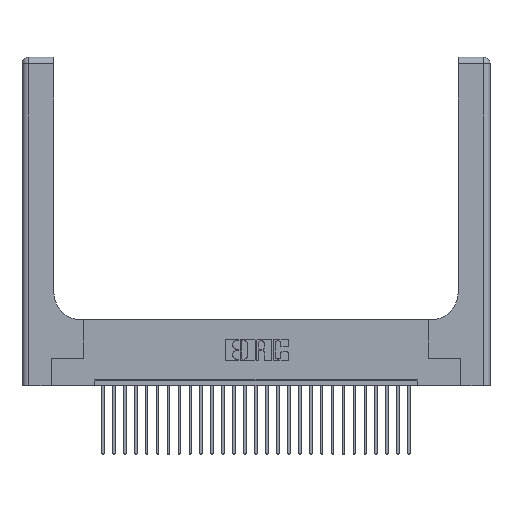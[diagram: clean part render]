
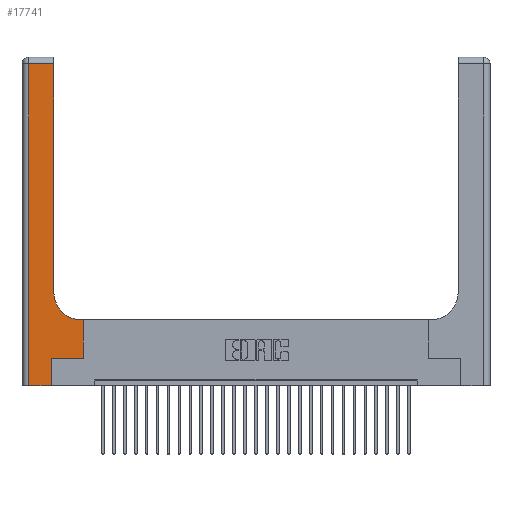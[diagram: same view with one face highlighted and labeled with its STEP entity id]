
A CAD part, top view. The second image highlights one B-rep face of the part: STEP entity #17741.
In plain terms, the highlighted planar face has unit normal (0, 0, 1).
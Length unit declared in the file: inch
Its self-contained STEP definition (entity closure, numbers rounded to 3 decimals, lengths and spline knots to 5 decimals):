
#417 = DIRECTION ( 'NONE',  ( -1., 0., 0. ) ) ;
#625 = PLANE ( 'NONE',  #6170 ) ;
#840 = CARTESIAN_POINT ( 'NONE',  ( 0.269, 0., 0.37 ) ) ;
#1347 = EDGE_LOOP ( 'NONE', ( #9175, #4184, #26375, #19203, #22407, #16420, #15048, #18807, #2289 ) ) ;
#1500 = AXIS2_PLACEMENT_3D ( 'NONE', #2193, #4414, #19921 ) ;
#2193 = CARTESIAN_POINT ( 'NONE',  ( 0.5415, 0.85, 0.37 ) ) ;
#2289 = ORIENTED_EDGE ( 'NONE', *, *, #15588, .T. ) ;
#2586 = CARTESIAN_POINT ( 'NONE',  ( 0.2915, 3., 0.37 ) ) ;
#2830 = VERTEX_POINT ( 'NONE', #20505 ) ;
#2966 = DIRECTION ( 'NONE',  ( 0., 1., 0. ) ) ;
#3234 = VECTOR ( 'NONE', #13790, 39.37008 ) ;
#3488 = VERTEX_POINT ( 'NONE', #12403 ) ;
#3917 = LINE ( 'NONE', #2586, #25105 ) ;
#4184 = ORIENTED_EDGE ( 'NONE', *, *, #13739, .T. ) ;
#4414 = DIRECTION ( 'NONE',  ( 0., 0., -1. ) ) ;
#4585 = CARTESIAN_POINT ( 'NONE',  ( 0.5585, 0.25, 0.37 ) ) ;
#4624 = VERTEX_POINT ( 'NONE', #21153 ) ;
#4930 = EDGE_CURVE ( 'NONE', #28707, #27301, #27246, .T. ) ;
#5754 = LINE ( 'NONE', #11233, #25561 ) ;
#6040 = CARTESIAN_POINT ( 'NONE',  ( 0., 2.94, 0.37 ) ) ;
#6170 = AXIS2_PLACEMENT_3D ( 'NONE', #9366, #20423, #417 ) ;
#6558 = CARTESIAN_POINT ( 'NONE',  ( 0.06, 0., 0.37 ) ) ;
#6717 = CARTESIAN_POINT ( 'NONE',  ( 0., 0., 0.37 ) ) ;
#6831 = CARTESIAN_POINT ( 'NONE',  ( 0.269, 0.25, 0.37 ) ) ;
#7034 = DIRECTION ( 'NONE',  ( 0., 1., 0. ) ) ;
#8429 = EDGE_CURVE ( 'NONE', #17625, #28707, #8473, .T. ) ;
#8473 = LINE ( 'NONE', #6717, #23761 ) ;
#8749 = CARTESIAN_POINT ( 'NONE',  ( 0.5585, 0.6, 0.37 ) ) ;
#9175 = ORIENTED_EDGE ( 'NONE', *, *, #24124, .T. ) ;
#9303 = CARTESIAN_POINT ( 'NONE',  ( 0.06, 3., 0.37 ) ) ;
#9366 = CARTESIAN_POINT ( 'NONE',  ( 0., 3., 0.37 ) ) ;
#9421 = LINE ( 'NONE', #28574, #18408 ) ;
#10050 = EDGE_CURVE ( 'NONE', #16948, #25199, #9421, .T. ) ;
#11233 = CARTESIAN_POINT ( 'NONE',  ( 0.2915, 0.6, 0.37 ) ) ;
#12403 = CARTESIAN_POINT ( 'NONE',  ( 0.5415, 0.6, 0.37 ) ) ;
#13149 = DIRECTION ( 'NONE',  ( 0., 1., 0. ) ) ;
#13739 = EDGE_CURVE ( 'NONE', #2830, #20720, #24396, .T. ) ;
#13790 = DIRECTION ( 'NONE',  ( 0., -1., 0. ) ) ;
#14092 = FACE_OUTER_BOUND ( 'NONE', #1347, .T. ) ;
#14741 = VECTOR ( 'NONE', #2966, 39.37008 ) ;
#15041 = LINE ( 'NONE', #9303, #3234 ) ;
#15048 = ORIENTED_EDGE ( 'NONE', *, *, #10050, .T. ) ;
#15588 = EDGE_CURVE ( 'NONE', #3488, #4624, #21570, .T. ) ;
#16420 = ORIENTED_EDGE ( 'NONE', *, *, #22112, .T. ) ;
#16948 = VERTEX_POINT ( 'NONE', #4585 ) ;
#17490 = LINE ( 'NONE', #23381, #23830 ) ;
#17625 = VERTEX_POINT ( 'NONE', #6558 ) ;
#17661 = EDGE_CURVE ( 'NONE', #25199, #3488, #5754, .T. ) ;
#17741 = ADVANCED_FACE ( 'NONE', ( #14092 ), #625, .F. ) ;
#18408 = VECTOR ( 'NONE', #13149, 39.37008 ) ;
#18807 = ORIENTED_EDGE ( 'NONE', *, *, #17661, .T. ) ;
#19203 = ORIENTED_EDGE ( 'NONE', *, *, #8429, .T. ) ;
#19921 = DIRECTION ( 'NONE',  ( 1., 0., 0. ) ) ;
#19938 = DIRECTION ( 'NONE',  ( -1., 0., 0. ) ) ;
#20423 = DIRECTION ( 'NONE',  ( 0., 0., -1. ) ) ;
#20505 = CARTESIAN_POINT ( 'NONE',  ( 0.2915, 2.94, 0.37 ) ) ;
#20720 = VERTEX_POINT ( 'NONE', #27943 ) ;
#21153 = CARTESIAN_POINT ( 'NONE',  ( 0.2915, 0.85, 0.37 ) ) ;
#21570 = CIRCLE ( 'NONE', #1500, 0.25 ) ;
#21800 = DIRECTION ( 'NONE',  ( -1., 0., 0. ) ) ;
#22112 = EDGE_CURVE ( 'NONE', #27301, #16948, #17490, .T. ) ;
#22407 = ORIENTED_EDGE ( 'NONE', *, *, #4930, .T. ) ;
#22576 = DIRECTION ( 'NONE',  ( 1., 0., 0. ) ) ;
#23381 = CARTESIAN_POINT ( 'NONE',  ( 0.269, 0.25, 0.37 ) ) ;
#23521 = EDGE_CURVE ( 'NONE', #20720, #17625, #15041, .T. ) ;
#23761 = VECTOR ( 'NONE', #22576, 39.37008 ) ;
#23830 = VECTOR ( 'NONE', #25384, 39.37008 ) ;
#24124 = EDGE_CURVE ( 'NONE', #4624, #2830, #3917, .T. ) ;
#24396 = LINE ( 'NONE', #6040, #27150 ) ;
#25105 = VECTOR ( 'NONE', #7034, 39.37008 ) ;
#25199 = VERTEX_POINT ( 'NONE', #8749 ) ;
#25384 = DIRECTION ( 'NONE',  ( 1., 0., 0. ) ) ;
#25561 = VECTOR ( 'NONE', #19938, 39.37008 ) ;
#26375 = ORIENTED_EDGE ( 'NONE', *, *, #23521, .T. ) ;
#27150 = VECTOR ( 'NONE', #21800, 39.37008 ) ;
#27246 = LINE ( 'NONE', #840, #14741 ) ;
#27301 = VERTEX_POINT ( 'NONE', #6831 ) ;
#27806 = CARTESIAN_POINT ( 'NONE',  ( 0.269, 0., 0.37 ) ) ;
#27943 = CARTESIAN_POINT ( 'NONE',  ( 0.06, 2.94, 0.37 ) ) ;
#28574 = CARTESIAN_POINT ( 'NONE',  ( 0.5585, 0.25, 0.37 ) ) ;
#28707 = VERTEX_POINT ( 'NONE', #27806 ) ;
